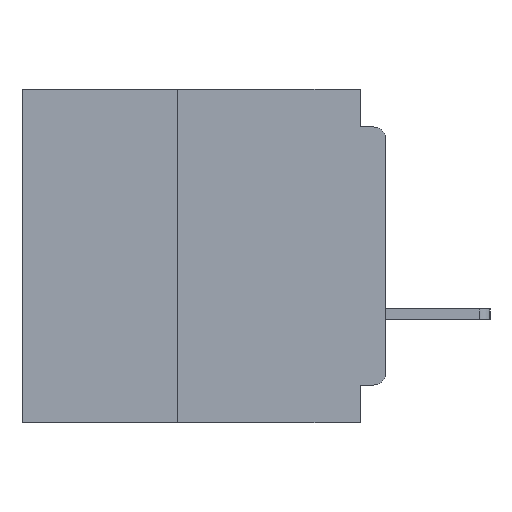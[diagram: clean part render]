
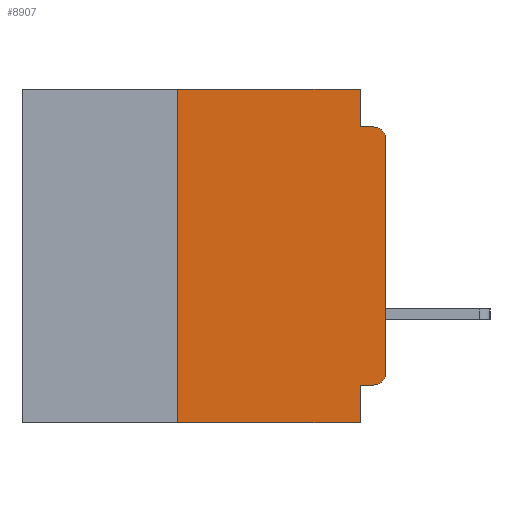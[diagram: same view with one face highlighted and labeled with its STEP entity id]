
A CAD part, left-side view. The second image highlights one B-rep face of the part: STEP entity #8907.
In plain terms, the highlighted planar face has unit normal (-1, 0, 0).
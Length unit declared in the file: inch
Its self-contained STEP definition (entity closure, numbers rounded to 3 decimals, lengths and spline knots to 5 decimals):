
#375 = VECTOR ( 'NONE', #15238, 39.37008 ) ;
#431 = EDGE_LOOP ( 'NONE', ( #33706, #28539, #30091, #7941, #16411, #24969, #26431, #16450, #11436, #28913 ) ) ;
#1064 = CARTESIAN_POINT ( 'NONE',  ( 0., 0.031, -0.4 ) ) ;
#1145 = VERTEX_POINT ( 'NONE', #12390 ) ;
#1315 = LINE ( 'NONE', #9668, #375 ) ;
#1654 = LINE ( 'NONE', #19402, #22794 ) ;
#1674 = EDGE_CURVE ( 'NONE', #18141, #9734, #17085, .T. ) ;
#1779 = VERTEX_POINT ( 'NONE', #30746 ) ;
#2708 = CARTESIAN_POINT ( 'NONE',  ( 0., 0.015, -0.06 ) ) ;
#3377 = VERTEX_POINT ( 'NONE', #7311 ) ;
#3954 = CARTESIAN_POINT ( 'NONE',  ( 0., 0., -0.06 ) ) ;
#5688 = DIRECTION ( 'NONE',  ( 0., 0., -1. ) ) ;
#6775 = EDGE_CURVE ( 'NONE', #36017, #11893, #33150, .T. ) ;
#7311 = CARTESIAN_POINT ( 'NONE',  ( 0., 0.25, 0. ) ) ;
#7941 = ORIENTED_EDGE ( 'NONE', *, *, #6775, .F. ) ;
#7963 = EDGE_CURVE ( 'NONE', #11893, #1145, #1315, .T. ) ;
#8200 = CARTESIAN_POINT ( 'NONE',  ( 0., 0.031, -0.045 ) ) ;
#8794 = EDGE_CURVE ( 'NONE', #29461, #18141, #18901, .T. ) ;
#8907 = ADVANCED_FACE ( 'NONE', ( #29529 ), #22407, .F. ) ;
#9009 = DIRECTION ( 'NONE',  ( -1., 0., 0. ) ) ;
#9294 = AXIS2_PLACEMENT_3D ( 'NONE', #2708, #22782, #5688 ) ;
#9532 = VECTOR ( 'NONE', #19255, 39.37008 ) ;
#9668 = CARTESIAN_POINT ( 'NONE',  ( 0., 0., -0.045 ) ) ;
#9734 = VERTEX_POINT ( 'NONE', #1064 ) ;
#10193 = EDGE_CURVE ( 'NONE', #29461, #25589, #23678, .T. ) ;
#10462 = VERTEX_POINT ( 'NONE', #3954 ) ;
#10680 = CARTESIAN_POINT ( 'NONE',  ( 0., 0.031, -0.4 ) ) ;
#10997 = AXIS2_PLACEMENT_3D ( 'NONE', #25980, #9009, #28836 ) ;
#11062 = CARTESIAN_POINT ( 'NONE',  ( 0., 0.437, -0.4 ) ) ;
#11085 = DIRECTION ( 'NONE',  ( 1., 0., 0. ) ) ;
#11436 = ORIENTED_EDGE ( 'NONE', *, *, #8794, .F. ) ;
#11893 = VERTEX_POINT ( 'NONE', #8200 ) ;
#12390 = CARTESIAN_POINT ( 'NONE',  ( 0., 0.015, -0.045 ) ) ;
#13984 = CIRCLE ( 'NONE', #9294, 0.015 ) ;
#14458 = EDGE_CURVE ( 'NONE', #1779, #3377, #1654, .T. ) ;
#15238 = DIRECTION ( 'NONE',  ( 0., -1., 0. ) ) ;
#16411 = ORIENTED_EDGE ( 'NONE', *, *, #18247, .F. ) ;
#16450 = ORIENTED_EDGE ( 'NONE', *, *, #1674, .F. ) ;
#16744 = CARTESIAN_POINT ( 'NONE',  ( 0., 0.031, 0. ) ) ;
#17085 = LINE ( 'NONE', #10680, #9532 ) ;
#17119 = VECTOR ( 'NONE', #36090, 39.37008 ) ;
#18141 = VERTEX_POINT ( 'NONE', #36707 ) ;
#18247 = EDGE_CURVE ( 'NONE', #3377, #36017, #30722, .T. ) ;
#18901 = LINE ( 'NONE', #27558, #17119 ) ;
#19255 = DIRECTION ( 'NONE',  ( 0., 0., -1. ) ) ;
#19402 = CARTESIAN_POINT ( 'NONE',  ( 0., 0.25, -0.4 ) ) ;
#19603 = DIRECTION ( 'NONE',  ( 0., 0., -1. ) ) ;
#22407 = PLANE ( 'NONE',  #24045 ) ;
#22782 = DIRECTION ( 'NONE',  ( -1., 0., 0. ) ) ;
#22794 = VECTOR ( 'NONE', #36212, 39.37008 ) ;
#23233 = VECTOR ( 'NONE', #28674, 39.37008 ) ;
#23678 = CIRCLE ( 'NONE', #10997, 0.015 ) ;
#24045 = AXIS2_PLACEMENT_3D ( 'NONE', #28058, #11085, #30908 ) ;
#24762 = VECTOR ( 'NONE', #19603, 39.37008 ) ;
#24969 = ORIENTED_EDGE ( 'NONE', *, *, #14458, .F. ) ;
#25589 = VERTEX_POINT ( 'NONE', #30152 ) ;
#25736 = EDGE_CURVE ( 'NONE', #1779, #9734, #26693, .T. ) ;
#25980 = CARTESIAN_POINT ( 'NONE',  ( 0., 0.015, -0.34 ) ) ;
#26431 = ORIENTED_EDGE ( 'NONE', *, *, #25736, .T. ) ;
#26693 = LINE ( 'NONE', #11062, #34217 ) ;
#26748 = EDGE_CURVE ( 'NONE', #25589, #10462, #28832, .T. ) ;
#26886 = CARTESIAN_POINT ( 'NONE',  ( 0., 0.015, -0.355 ) ) ;
#27558 = CARTESIAN_POINT ( 'NONE',  ( 0., 0., -0.355 ) ) ;
#28058 = CARTESIAN_POINT ( 'NONE',  ( 0., 0.437, 0. ) ) ;
#28539 = ORIENTED_EDGE ( 'NONE', *, *, #35456, .T. ) ;
#28674 = DIRECTION ( 'NONE',  ( 0., -1., 0. ) ) ;
#28832 = LINE ( 'NONE', #30431, #34580 ) ;
#28836 = DIRECTION ( 'NONE',  ( 0., 0., -1. ) ) ;
#28913 = ORIENTED_EDGE ( 'NONE', *, *, #10193, .T. ) ;
#29461 = VERTEX_POINT ( 'NONE', #26886 ) ;
#29529 = FACE_OUTER_BOUND ( 'NONE', #431, .T. ) ;
#30091 = ORIENTED_EDGE ( 'NONE', *, *, #7963, .F. ) ;
#30152 = CARTESIAN_POINT ( 'NONE',  ( 0., 0., -0.34 ) ) ;
#30431 = CARTESIAN_POINT ( 'NONE',  ( 0., 0., 0. ) ) ;
#30722 = LINE ( 'NONE', #31403, #23233 ) ;
#30746 = CARTESIAN_POINT ( 'NONE',  ( 0., 0.25, -0.4 ) ) ;
#30908 = DIRECTION ( 'NONE',  ( 0., 0., -1. ) ) ;
#31403 = CARTESIAN_POINT ( 'NONE',  ( 0., 0.437, 0. ) ) ;
#33150 = LINE ( 'NONE', #16744, #24762 ) ;
#33276 = DIRECTION ( 'NONE',  ( 0., 0., 1. ) ) ;
#33706 = ORIENTED_EDGE ( 'NONE', *, *, #26748, .T. ) ;
#33715 = DIRECTION ( 'NONE',  ( 0., -1., 0. ) ) ;
#34217 = VECTOR ( 'NONE', #33715, 39.37008 ) ;
#34580 = VECTOR ( 'NONE', #33276, 39.37008 ) ;
#35456 = EDGE_CURVE ( 'NONE', #10462, #1145, #13984, .T. ) ;
#35580 = CARTESIAN_POINT ( 'NONE',  ( 0., 0.031, 0. ) ) ;
#36017 = VERTEX_POINT ( 'NONE', #35580 ) ;
#36090 = DIRECTION ( 'NONE',  ( 0., 1., 0. ) ) ;
#36212 = DIRECTION ( 'NONE',  ( 0., 0., 1. ) ) ;
#36707 = CARTESIAN_POINT ( 'NONE',  ( 0., 0.031, -0.355 ) ) ;
